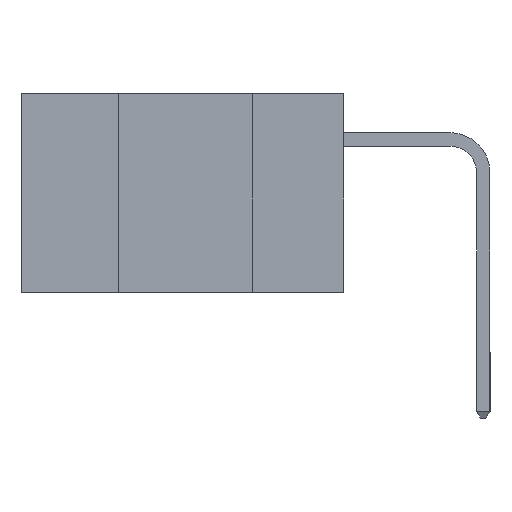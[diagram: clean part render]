
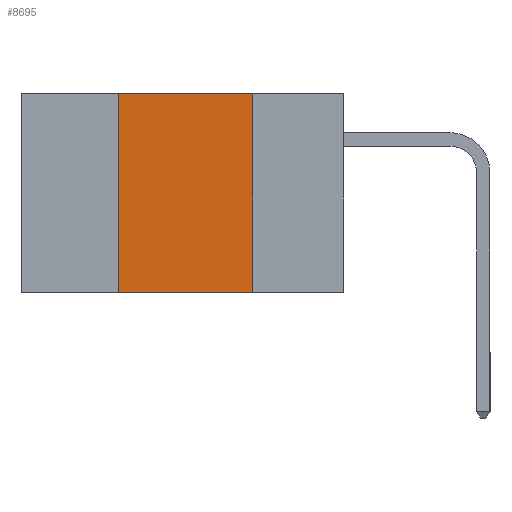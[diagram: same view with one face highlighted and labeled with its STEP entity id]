
A CAD part, left-side view. The second image highlights one B-rep face of the part: STEP entity #8695.
In plain terms, the highlighted planar face has unit normal (-1, 0, 0).
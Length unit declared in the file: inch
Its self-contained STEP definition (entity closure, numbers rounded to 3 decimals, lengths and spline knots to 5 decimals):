
#56 = ORIENTED_EDGE ( 'NONE', *, *, #6570, .F. ) ;
#728 = VERTEX_POINT ( 'NONE', #3173 ) ;
#885 = CARTESIAN_POINT ( 'NONE',  ( 0., 0.42, 0. ) ) ;
#1172 = EDGE_CURVE ( 'NONE', #3691, #10970, #16696, .T. ) ;
#1703 = VERTEX_POINT ( 'NONE', #885 ) ;
#2621 = AXIS2_PLACEMENT_3D ( 'NONE', #8841, #12731, #15362 ) ;
#2885 = CARTESIAN_POINT ( 'NONE',  ( 0., 0.6, -0.37 ) ) ;
#2995 = CARTESIAN_POINT ( 'NONE',  ( 0., 0.17, 0. ) ) ;
#3173 = CARTESIAN_POINT ( 'NONE',  ( 0., 0.42, -0.37 ) ) ;
#3691 = VERTEX_POINT ( 'NONE', #2995 ) ;
#4407 = ORIENTED_EDGE ( 'NONE', *, *, #15259, .F. ) ;
#6083 = ORIENTED_EDGE ( 'NONE', *, *, #9239, .T. ) ;
#6570 = EDGE_CURVE ( 'NONE', #1703, #3691, #9214, .T. ) ;
#6936 = ORIENTED_EDGE ( 'NONE', *, *, #1172, .F. ) ;
#8695 = ADVANCED_FACE ( 'NONE', ( #9349 ), #11418, .F. ) ;
#8841 = CARTESIAN_POINT ( 'NONE',  ( 0., 0.6, 0. ) ) ;
#9214 = LINE ( 'NONE', #16586, #9844 ) ;
#9239 = EDGE_CURVE ( 'NONE', #728, #10970, #16439, .T. ) ;
#9334 = VECTOR ( 'NONE', #10965, 39.37008 ) ;
#9349 = FACE_OUTER_BOUND ( 'NONE', #14161, .T. ) ;
#9632 = DIRECTION ( 'NONE',  ( 0., -1., 0. ) ) ;
#9844 = VECTOR ( 'NONE', #9632, 39.37008 ) ;
#10609 = CARTESIAN_POINT ( 'NONE',  ( 0., 0.17, 0. ) ) ;
#10683 = VECTOR ( 'NONE', #14899, 39.37008 ) ;
#10767 = CARTESIAN_POINT ( 'NONE',  ( 0., 0.42, 0. ) ) ;
#10965 = DIRECTION ( 'NONE',  ( 0., -1., 0. ) ) ;
#10970 = VERTEX_POINT ( 'NONE', #15137 ) ;
#11418 = PLANE ( 'NONE',  #2621 ) ;
#11836 = DIRECTION ( 'NONE',  ( 0., 0., -1. ) ) ;
#12731 = DIRECTION ( 'NONE',  ( 1., 0., 0. ) ) ;
#13800 = LINE ( 'NONE', #10767, #10683 ) ;
#14161 = EDGE_LOOP ( 'NONE', ( #6936, #56, #4407, #6083 ) ) ;
#14899 = DIRECTION ( 'NONE',  ( 0., 0., 1. ) ) ;
#15137 = CARTESIAN_POINT ( 'NONE',  ( 0., 0.17, -0.37 ) ) ;
#15259 = EDGE_CURVE ( 'NONE', #728, #1703, #13800, .T. ) ;
#15362 = DIRECTION ( 'NONE',  ( 0., 0., -1. ) ) ;
#16051 = VECTOR ( 'NONE', #11836, 39.37008 ) ;
#16439 = LINE ( 'NONE', #2885, #9334 ) ;
#16586 = CARTESIAN_POINT ( 'NONE',  ( 0., 0.6, 0. ) ) ;
#16696 = LINE ( 'NONE', #10609, #16051 ) ;
